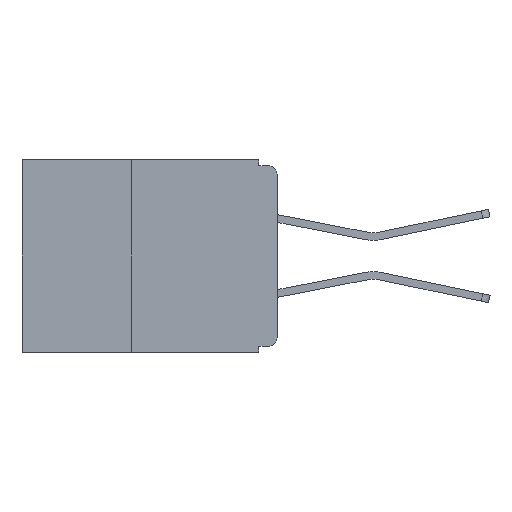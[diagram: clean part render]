
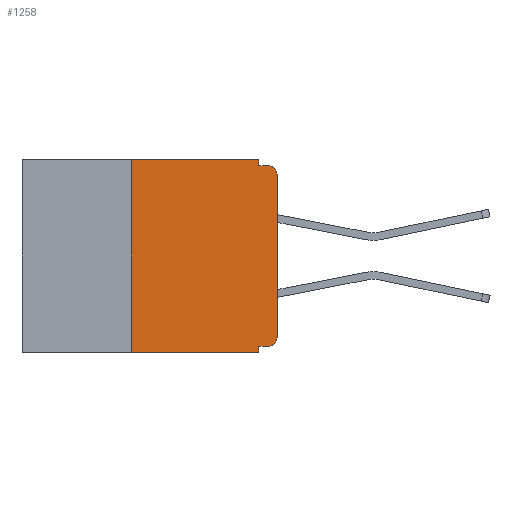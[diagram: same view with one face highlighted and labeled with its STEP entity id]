
A CAD part, left-side view. The second image highlights one B-rep face of the part: STEP entity #1258.
In plain terms, the highlighted planar face has unit normal (-1, 0, 0).
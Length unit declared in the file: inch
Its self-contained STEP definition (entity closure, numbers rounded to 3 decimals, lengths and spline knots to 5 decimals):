
#428 = CIRCLE ( 'NONE', #4223, 0.015 ) ;
#577 = LINE ( 'NONE', #7290, #7162 ) ;
#593 = VERTEX_POINT ( 'NONE', #13062 ) ;
#1000 = ORIENTED_EDGE ( 'NONE', *, *, #13182, .F. ) ;
#1258 = ADVANCED_FACE ( 'NONE', ( #6978 ), #12013, .F. ) ;
#1287 = ORIENTED_EDGE ( 'NONE', *, *, #6649, .F. ) ;
#1364 = DIRECTION ( 'NONE',  ( 0., 0., 1. ) ) ;
#1395 = VERTEX_POINT ( 'NONE', #3116 ) ;
#1464 = DIRECTION ( 'NONE',  ( 0., 0., -1. ) ) ;
#1846 = EDGE_CURVE ( 'NONE', #2584, #12838, #15706, .T. ) ;
#1979 = VECTOR ( 'NONE', #4115, 39.37008 ) ;
#2584 = VERTEX_POINT ( 'NONE', #8274 ) ;
#2663 = AXIS2_PLACEMENT_3D ( 'NONE', #12818, #11824, #11764 ) ;
#2876 = LINE ( 'NONE', #11157, #9029 ) ;
#2890 = AXIS2_PLACEMENT_3D ( 'NONE', #8147, #14496, #11668 ) ;
#3116 = CARTESIAN_POINT ( 'NONE',  ( 0., 0.031, -0.33 ) ) ;
#3384 = CARTESIAN_POINT ( 'NONE',  ( 0., 0.031, -0.01 ) ) ;
#3559 = CARTESIAN_POINT ( 'NONE',  ( 0., 0., -0.01 ) ) ;
#3916 = ORIENTED_EDGE ( 'NONE', *, *, #13419, .F. ) ;
#4066 = VECTOR ( 'NONE', #15905, 39.37008 ) ;
#4115 = DIRECTION ( 'NONE',  ( 0., 0., 1. ) ) ;
#4187 = ORIENTED_EDGE ( 'NONE', *, *, #7198, .T. ) ;
#4223 = AXIS2_PLACEMENT_3D ( 'NONE', #16169, #16111, #15939 ) ;
#4855 = DIRECTION ( 'NONE',  ( 0., -1., 0. ) ) ;
#5248 = EDGE_CURVE ( 'NONE', #6373, #13824, #428, .T. ) ;
#5304 = CARTESIAN_POINT ( 'NONE',  ( 0., 0.031, 0. ) ) ;
#5392 = EDGE_CURVE ( 'NONE', #6245, #8056, #8054, .T. ) ;
#5711 = VECTOR ( 'NONE', #1464, 39.37008 ) ;
#5815 = DIRECTION ( 'NONE',  ( 0., -1., 0. ) ) ;
#5883 = CARTESIAN_POINT ( 'NONE',  ( 0., 0.437, 0. ) ) ;
#6245 = VERTEX_POINT ( 'NONE', #13248 ) ;
#6373 = VERTEX_POINT ( 'NONE', #13515 ) ;
#6649 = EDGE_CURVE ( 'NONE', #11572, #13824, #13550, .T. ) ;
#6978 = FACE_OUTER_BOUND ( 'NONE', #13142, .T. ) ;
#7147 = VERTEX_POINT ( 'NONE', #8513 ) ;
#7162 = VECTOR ( 'NONE', #7349, 39.37008 ) ;
#7198 = EDGE_CURVE ( 'NONE', #7147, #1395, #577, .T. ) ;
#7290 = CARTESIAN_POINT ( 'NONE',  ( 0., 0.437, -0.33 ) ) ;
#7349 = DIRECTION ( 'NONE',  ( 0., -1., 0. ) ) ;
#7556 = LINE ( 'NONE', #10754, #4066 ) ;
#8054 = LINE ( 'NONE', #5883, #14989 ) ;
#8056 = VERTEX_POINT ( 'NONE', #5304 ) ;
#8147 = CARTESIAN_POINT ( 'NONE',  ( 0., 0.015, -0.305 ) ) ;
#8274 = CARTESIAN_POINT ( 'NONE',  ( 0., 0.015, -0.32 ) ) ;
#8322 = ORIENTED_EDGE ( 'NONE', *, *, #1846, .T. ) ;
#8513 = CARTESIAN_POINT ( 'NONE',  ( 0., 0.25, -0.33 ) ) ;
#8807 = ORIENTED_EDGE ( 'NONE', *, *, #15552, .T. ) ;
#9029 = VECTOR ( 'NONE', #9849, 39.37008 ) ;
#9095 = LINE ( 'NONE', #16915, #12981 ) ;
#9246 = LINE ( 'NONE', #13231, #5711 ) ;
#9610 = CARTESIAN_POINT ( 'NONE',  ( 0., 0.015, -0.01 ) ) ;
#9849 = DIRECTION ( 'NONE',  ( 0., 0., -1. ) ) ;
#10754 = CARTESIAN_POINT ( 'NONE',  ( 0., 0., -0.32 ) ) ;
#10970 = EDGE_CURVE ( 'NONE', #7147, #6245, #9095, .T. ) ;
#11157 = CARTESIAN_POINT ( 'NONE',  ( 0., 0.031, -0.33 ) ) ;
#11285 = ORIENTED_EDGE ( 'NONE', *, *, #5248, .T. ) ;
#11572 = VERTEX_POINT ( 'NONE', #3384 ) ;
#11668 = DIRECTION ( 'NONE',  ( 0., 0., -1. ) ) ;
#11764 = DIRECTION ( 'NONE',  ( 0., 0., -1. ) ) ;
#11824 = DIRECTION ( 'NONE',  ( 1., 0., 0. ) ) ;
#11979 = CARTESIAN_POINT ( 'NONE',  ( 0., 0., 0. ) ) ;
#12008 = LINE ( 'NONE', #11979, #1979 ) ;
#12013 = PLANE ( 'NONE',  #2663 ) ;
#12762 = VECTOR ( 'NONE', #4855, 39.37008 ) ;
#12818 = CARTESIAN_POINT ( 'NONE',  ( 0., 0.437, 0. ) ) ;
#12838 = VERTEX_POINT ( 'NONE', #13805 ) ;
#12981 = VECTOR ( 'NONE', #1364, 39.37008 ) ;
#13062 = CARTESIAN_POINT ( 'NONE',  ( 0., 0.031, -0.32 ) ) ;
#13142 = EDGE_LOOP ( 'NONE', ( #8807, #11285, #1287, #1000, #15268, #15522, #4187, #3916, #13442, #8322 ) ) ;
#13182 = EDGE_CURVE ( 'NONE', #8056, #11572, #9246, .T. ) ;
#13231 = CARTESIAN_POINT ( 'NONE',  ( 0., 0.031, 0. ) ) ;
#13248 = CARTESIAN_POINT ( 'NONE',  ( 0., 0.25, 0. ) ) ;
#13419 = EDGE_CURVE ( 'NONE', #593, #1395, #2876, .T. ) ;
#13442 = ORIENTED_EDGE ( 'NONE', *, *, #13737, .F. ) ;
#13515 = CARTESIAN_POINT ( 'NONE',  ( 0., 0., -0.025 ) ) ;
#13550 = LINE ( 'NONE', #3559, #12762 ) ;
#13737 = EDGE_CURVE ( 'NONE', #2584, #593, #7556, .T. ) ;
#13805 = CARTESIAN_POINT ( 'NONE',  ( 0., 0., -0.305 ) ) ;
#13824 = VERTEX_POINT ( 'NONE', #9610 ) ;
#14496 = DIRECTION ( 'NONE',  ( -1., 0., 0. ) ) ;
#14989 = VECTOR ( 'NONE', #5815, 39.37008 ) ;
#15268 = ORIENTED_EDGE ( 'NONE', *, *, #5392, .F. ) ;
#15522 = ORIENTED_EDGE ( 'NONE', *, *, #10970, .F. ) ;
#15552 = EDGE_CURVE ( 'NONE', #12838, #6373, #12008, .T. ) ;
#15706 = CIRCLE ( 'NONE', #2890, 0.015 ) ;
#15905 = DIRECTION ( 'NONE',  ( 0., 1., 0. ) ) ;
#15939 = DIRECTION ( 'NONE',  ( 0., 0., -1. ) ) ;
#16111 = DIRECTION ( 'NONE',  ( -1., 0., 0. ) ) ;
#16169 = CARTESIAN_POINT ( 'NONE',  ( 0., 0.015, -0.025 ) ) ;
#16915 = CARTESIAN_POINT ( 'NONE',  ( 0., 0.25, -0.33 ) ) ;
